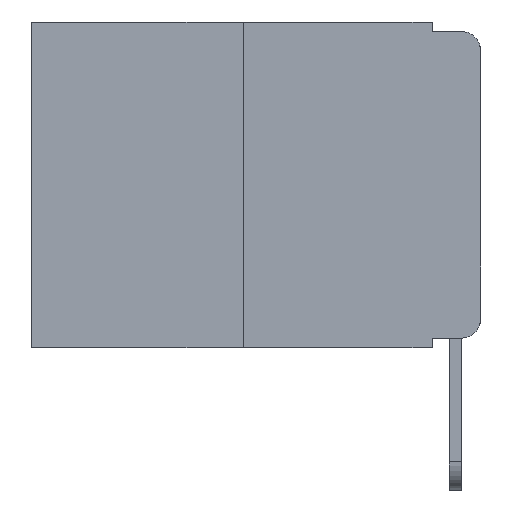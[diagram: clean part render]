
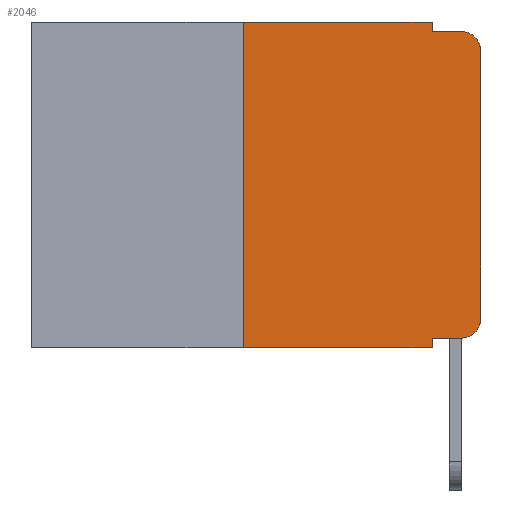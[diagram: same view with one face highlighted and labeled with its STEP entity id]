
A CAD part, left-side view. The second image highlights one B-rep face of the part: STEP entity #2046.
In plain terms, the highlighted planar face has unit normal (-1, 0, 0).
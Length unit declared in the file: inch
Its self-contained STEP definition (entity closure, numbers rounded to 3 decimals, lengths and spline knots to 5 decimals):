
#53 = CARTESIAN_POINT ( 'NONE',  ( 0., 0., 0. ) ) ;
#363 = CARTESIAN_POINT ( 'NONE',  ( 0., 0., -0.313 ) ) ;
#482 = CARTESIAN_POINT ( 'NONE',  ( 0., 0.051, 0. ) ) ;
#559 = EDGE_CURVE ( 'NONE', #6785, #8807, #15456, .T. ) ;
#924 = EDGE_CURVE ( 'NONE', #1197, #7819, #15060, .T. ) ;
#952 = EDGE_CURVE ( 'NONE', #7819, #13119, #17633, .T. ) ;
#960 = EDGE_CURVE ( 'NONE', #9248, #13119, #8041, .T. ) ;
#989 = EDGE_CURVE ( 'NONE', #15954, #9248, #14695, .T. ) ;
#991 = EDGE_CURVE ( 'NONE', #6785, #17248, #17170, .T. ) ;
#1090 = EDGE_CURVE ( 'NONE', #16252, #8807, #16012, .T. ) ;
#1193 = DIRECTION ( 'NONE',  ( 0., -1., 0. ) ) ;
#1197 = VERTEX_POINT ( 'NONE', #363 ) ;
#1291 = CARTESIAN_POINT ( 'NONE',  ( 0., 0.051, -0.01 ) ) ;
#1294 = VERTEX_POINT ( 'NONE', #7869 ) ;
#1362 = EDGE_CURVE ( 'NONE', #16252, #1294, #2382, .T. ) ;
#1395 = EDGE_CURVE ( 'NONE', #1294, #1197, #10017, .T. ) ;
#1907 = ORIENTED_EDGE ( 'NONE', *, *, #1395, .T. ) ;
#2046 = ADVANCED_FACE ( 'NONE', ( #9126 ), #16470, .F. ) ;
#2109 = DIRECTION ( 'NONE',  ( -1., 0., 0. ) ) ;
#2236 = CARTESIAN_POINT ( 'NONE',  ( 0., 0.02, -0.03 ) ) ;
#2382 = LINE ( 'NONE', #11161, #17574 ) ;
#2718 = ORIENTED_EDGE ( 'NONE', *, *, #924, .T. ) ;
#3451 = DIRECTION ( 'NONE',  ( 0., 0., -1. ) ) ;
#3633 = CARTESIAN_POINT ( 'NONE',  ( 0., 0.02, -0.313 ) ) ;
#4016 = CARTESIAN_POINT ( 'NONE',  ( 0., 0., -0.03 ) ) ;
#4167 = DIRECTION ( 'NONE',  ( 1., 0., 0. ) ) ;
#4382 = CARTESIAN_POINT ( 'NONE',  ( 0., 0.051, 0. ) ) ;
#5259 = ORIENTED_EDGE ( 'NONE', *, *, #991, .F. ) ;
#5593 = AXIS2_PLACEMENT_3D ( 'NONE', #2236, #8543, #8404 ) ;
#6285 = DIRECTION ( 'NONE',  ( 0., 0., 1. ) ) ;
#6332 = CARTESIAN_POINT ( 'NONE',  ( 0., 0.25, 0. ) ) ;
#6785 = VERTEX_POINT ( 'NONE', #10478 ) ;
#6902 = DIRECTION ( 'NONE',  ( 0., 0., -1. ) ) ;
#6956 = ORIENTED_EDGE ( 'NONE', *, *, #952, .T. ) ;
#7117 = VECTOR ( 'NONE', #8750, 39.37008 ) ;
#7415 = DIRECTION ( 'NONE',  ( 0., -1., 0. ) ) ;
#7606 = CARTESIAN_POINT ( 'NONE',  ( 0., 0.02, -0.01 ) ) ;
#7819 = VERTEX_POINT ( 'NONE', #4016 ) ;
#7869 = CARTESIAN_POINT ( 'NONE',  ( 0., 0.02, -0.333 ) ) ;
#8041 = LINE ( 'NONE', #10055, #11227 ) ;
#8327 = ORIENTED_EDGE ( 'NONE', *, *, #989, .F. ) ;
#8404 = DIRECTION ( 'NONE',  ( 0., 0., -1. ) ) ;
#8543 = DIRECTION ( 'NONE',  ( -1., 0., 0. ) ) ;
#8750 = DIRECTION ( 'NONE',  ( 0., 0., 1. ) ) ;
#8807 = VERTEX_POINT ( 'NONE', #13087 ) ;
#8968 = DIRECTION ( 'NONE',  ( 0., 0., -1. ) ) ;
#9041 = CARTESIAN_POINT ( 'NONE',  ( 0., 0.051, -0.333 ) ) ;
#9126 = FACE_OUTER_BOUND ( 'NONE', #12087, .T. ) ;
#9220 = ORIENTED_EDGE ( 'NONE', *, *, #559, .T. ) ;
#9248 = VERTEX_POINT ( 'NONE', #1291 ) ;
#10017 = CIRCLE ( 'NONE', #15298, 0.02 ) ;
#10055 = CARTESIAN_POINT ( 'NONE',  ( 0., 0.051, -0.01 ) ) ;
#10388 = VECTOR ( 'NONE', #16548, 39.37008 ) ;
#10415 = VECTOR ( 'NONE', #8968, 39.37008 ) ;
#10478 = CARTESIAN_POINT ( 'NONE',  ( 0., 0.25, -0.343 ) ) ;
#11161 = CARTESIAN_POINT ( 'NONE',  ( 0., 0.051, -0.333 ) ) ;
#11227 = VECTOR ( 'NONE', #7415, 39.37008 ) ;
#11507 = CARTESIAN_POINT ( 'NONE',  ( 0., 0.473, 0. ) ) ;
#11679 = AXIS2_PLACEMENT_3D ( 'NONE', #17695, #4167, #14058 ) ;
#12087 = EDGE_LOOP ( 'NONE', ( #2718, #6956, #17803, #8327, #15312, #5259, #9220, #16079, #13166, #1907 ) ) ;
#13087 = CARTESIAN_POINT ( 'NONE',  ( 0., 0.051, -0.343 ) ) ;
#13119 = VERTEX_POINT ( 'NONE', #7606 ) ;
#13166 = ORIENTED_EDGE ( 'NONE', *, *, #1362, .T. ) ;
#14058 = DIRECTION ( 'NONE',  ( 0., 0., -1. ) ) ;
#14314 = CARTESIAN_POINT ( 'NONE',  ( 0., 0.25, 0. ) ) ;
#14695 = LINE ( 'NONE', #482, #10415 ) ;
#15060 = LINE ( 'NONE', #53, #15831 ) ;
#15205 = CARTESIAN_POINT ( 'NONE',  ( 0., 0.473, -0.343 ) ) ;
#15298 = AXIS2_PLACEMENT_3D ( 'NONE', #3633, #2109, #6902 ) ;
#15312 = ORIENTED_EDGE ( 'NONE', *, *, #16067, .F. ) ;
#15358 = DIRECTION ( 'NONE',  ( 0., -1., 0. ) ) ;
#15456 = LINE ( 'NONE', #15205, #15841 ) ;
#15831 = VECTOR ( 'NONE', #6285, 39.37008 ) ;
#15841 = VECTOR ( 'NONE', #15358, 39.37008 ) ;
#15954 = VERTEX_POINT ( 'NONE', #17674 ) ;
#16012 = LINE ( 'NONE', #4382, #16401 ) ;
#16067 = EDGE_CURVE ( 'NONE', #17248, #15954, #17139, .T. ) ;
#16079 = ORIENTED_EDGE ( 'NONE', *, *, #1090, .F. ) ;
#16252 = VERTEX_POINT ( 'NONE', #9041 ) ;
#16401 = VECTOR ( 'NONE', #3451, 39.37008 ) ;
#16470 = PLANE ( 'NONE',  #11679 ) ;
#16548 = DIRECTION ( 'NONE',  ( 0., -1., 0. ) ) ;
#17139 = LINE ( 'NONE', #11507, #10388 ) ;
#17170 = LINE ( 'NONE', #6332, #7117 ) ;
#17248 = VERTEX_POINT ( 'NONE', #14314 ) ;
#17574 = VECTOR ( 'NONE', #1193, 39.37008 ) ;
#17633 = CIRCLE ( 'NONE', #5593, 0.02 ) ;
#17674 = CARTESIAN_POINT ( 'NONE',  ( 0., 0.051, 0. ) ) ;
#17695 = CARTESIAN_POINT ( 'NONE',  ( 0., 0.473, 0. ) ) ;
#17803 = ORIENTED_EDGE ( 'NONE', *, *, #960, .F. ) ;
